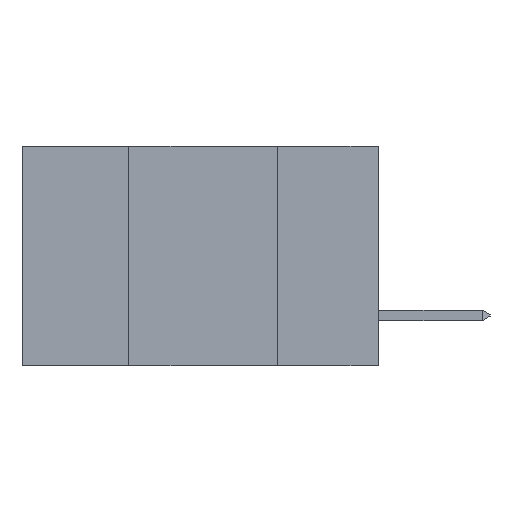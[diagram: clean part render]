
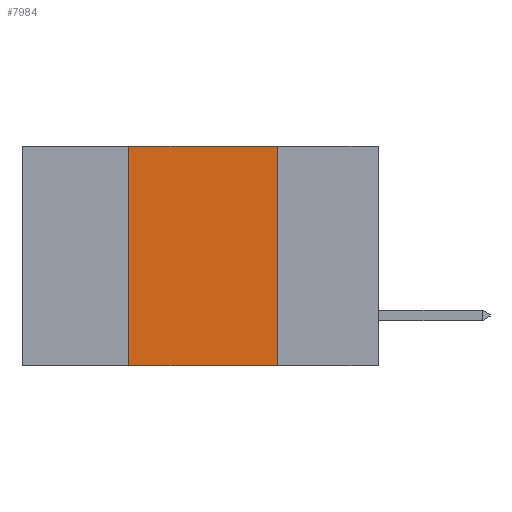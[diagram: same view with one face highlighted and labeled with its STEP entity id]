
A CAD part, left-side view. The second image highlights one B-rep face of the part: STEP entity #7984.
In plain terms, the highlighted planar face has unit normal (-1, 0, 0).
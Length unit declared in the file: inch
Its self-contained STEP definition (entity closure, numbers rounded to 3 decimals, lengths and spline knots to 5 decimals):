
#846 = VECTOR ( 'NONE', #1344, 39.37008 ) ;
#1088 = DIRECTION ( 'NONE',  ( 0., 0., 1. ) ) ;
#1320 = ORIENTED_EDGE ( 'NONE', *, *, #3567, .F. ) ;
#1344 = DIRECTION ( 'NONE',  ( 0., 0., -1. ) ) ;
#1919 = LINE ( 'NONE', #6975, #3987 ) ;
#2061 = VECTOR ( 'NONE', #5486, 39.37008 ) ;
#2256 = LINE ( 'NONE', #7198, #11163 ) ;
#2429 = DIRECTION ( 'NONE',  ( 0., 0., -1. ) ) ;
#2595 = LINE ( 'NONE', #7837, #2061 ) ;
#2659 = FACE_OUTER_BOUND ( 'NONE', #7568, .T. ) ;
#3567 = EDGE_CURVE ( 'NONE', #5988, #7157, #9839, .T. ) ;
#3627 = VERTEX_POINT ( 'NONE', #7701 ) ;
#3987 = VECTOR ( 'NONE', #7347, 39.37008 ) ;
#4223 = CARTESIAN_POINT ( 'NONE',  ( 0., 0.42, -0.37 ) ) ;
#4401 = EDGE_CURVE ( 'NONE', #6110, #7157, #1919, .T. ) ;
#4576 = EDGE_CURVE ( 'NONE', #3627, #5988, #2595, .T. ) ;
#5029 = CARTESIAN_POINT ( 'NONE',  ( 0., 0.6, 0. ) ) ;
#5486 = DIRECTION ( 'NONE',  ( 0., -1., 0. ) ) ;
#5858 = PLANE ( 'NONE',  #10659 ) ;
#5941 = ORIENTED_EDGE ( 'NONE', *, *, #4576, .F. ) ;
#5988 = VERTEX_POINT ( 'NONE', #10936 ) ;
#6110 = VERTEX_POINT ( 'NONE', #4223 ) ;
#6219 = ORIENTED_EDGE ( 'NONE', *, *, #8247, .F. ) ;
#6975 = CARTESIAN_POINT ( 'NONE',  ( 0., 0.6, -0.37 ) ) ;
#6988 = CARTESIAN_POINT ( 'NONE',  ( 0., 0.17, 0. ) ) ;
#7157 = VERTEX_POINT ( 'NONE', #7579 ) ;
#7198 = CARTESIAN_POINT ( 'NONE',  ( 0., 0.42, 0. ) ) ;
#7347 = DIRECTION ( 'NONE',  ( 0., -1., 0. ) ) ;
#7568 = EDGE_LOOP ( 'NONE', ( #1320, #5941, #6219, #10781 ) ) ;
#7579 = CARTESIAN_POINT ( 'NONE',  ( 0., 0.17, -0.37 ) ) ;
#7701 = CARTESIAN_POINT ( 'NONE',  ( 0., 0.42, 0. ) ) ;
#7703 = DIRECTION ( 'NONE',  ( 1., 0., 0. ) ) ;
#7837 = CARTESIAN_POINT ( 'NONE',  ( 0., 0.6, 0. ) ) ;
#7984 = ADVANCED_FACE ( 'NONE', ( #2659 ), #5858, .F. ) ;
#8247 = EDGE_CURVE ( 'NONE', #6110, #3627, #2256, .T. ) ;
#9839 = LINE ( 'NONE', #6988, #846 ) ;
#10659 = AXIS2_PLACEMENT_3D ( 'NONE', #5029, #7703, #2429 ) ;
#10781 = ORIENTED_EDGE ( 'NONE', *, *, #4401, .T. ) ;
#10936 = CARTESIAN_POINT ( 'NONE',  ( 0., 0.17, 0. ) ) ;
#11163 = VECTOR ( 'NONE', #1088, 39.37008 ) ;
